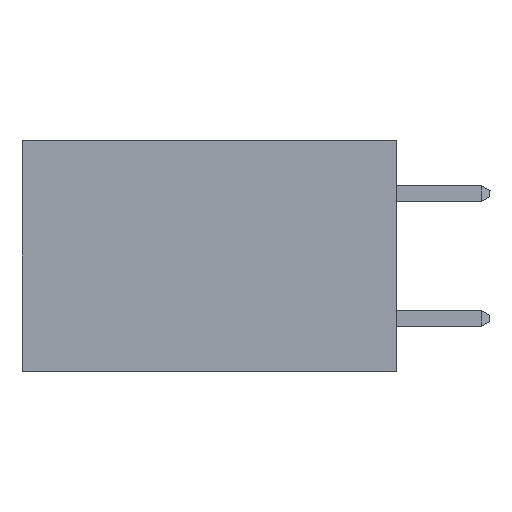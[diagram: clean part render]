
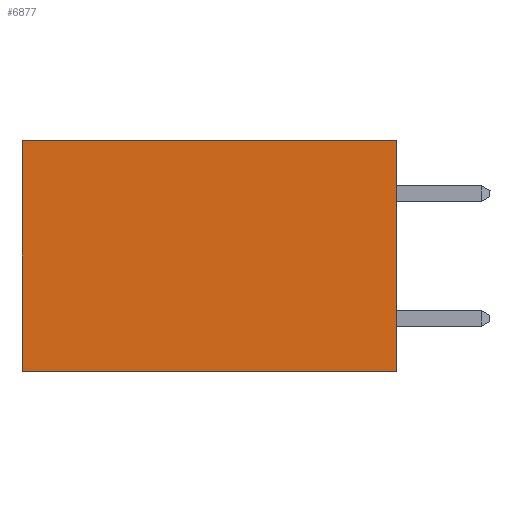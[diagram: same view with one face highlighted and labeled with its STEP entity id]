
A CAD part, left-side view. The second image highlights one B-rep face of the part: STEP entity #6877.
In plain terms, the highlighted planar face has unit normal (-1, 0, 0).
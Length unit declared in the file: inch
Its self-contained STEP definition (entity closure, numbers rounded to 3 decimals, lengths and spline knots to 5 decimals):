
#587 = VECTOR ( 'NONE', #7945, 39.37008 ) ;
#888 = CARTESIAN_POINT ( 'NONE',  ( 0.298, 0., 0. ) ) ;
#1716 = EDGE_CURVE ( 'NONE', #7474, #4993, #7250, .T. ) ;
#2394 = LINE ( 'NONE', #888, #11599 ) ;
#2653 = CARTESIAN_POINT ( 'NONE',  ( 0.298, 0.6, 0. ) ) ;
#3025 = ORIENTED_EDGE ( 'NONE', *, *, #7751, .F. ) ;
#4807 = LINE ( 'NONE', #15001, #8290 ) ;
#4993 = VERTEX_POINT ( 'NONE', #13291 ) ;
#5114 = ORIENTED_EDGE ( 'NONE', *, *, #14596, .F. ) ;
#5554 = DIRECTION ( 'NONE',  ( 0., 1., 0. ) ) ;
#6101 = VERTEX_POINT ( 'NONE', #13336 ) ;
#6487 = DIRECTION ( 'NONE',  ( 0., 1., 0. ) ) ;
#6577 = VERTEX_POINT ( 'NONE', #14257 ) ;
#6877 = ADVANCED_FACE ( 'NONE', ( #13568 ), #10319, .F. ) ;
#7250 = LINE ( 'NONE', #10048, #587 ) ;
#7474 = VERTEX_POINT ( 'NONE', #2653 ) ;
#7751 = EDGE_CURVE ( 'NONE', #6101, #4993, #9811, .T. ) ;
#7945 = DIRECTION ( 'NONE',  ( 0., 0., -1. ) ) ;
#8290 = VECTOR ( 'NONE', #6487, 39.37008 ) ;
#8355 = EDGE_CURVE ( 'NONE', #6577, #7474, #4807, .T. ) ;
#8827 = AXIS2_PLACEMENT_3D ( 'NONE', #10637, #10237, #10155 ) ;
#9141 = DIRECTION ( 'NONE',  ( 0., 0., -1. ) ) ;
#9811 = LINE ( 'NONE', #12825, #13152 ) ;
#10048 = CARTESIAN_POINT ( 'NONE',  ( 0.298, 0.6, 0. ) ) ;
#10155 = DIRECTION ( 'NONE',  ( 0., 0., -1. ) ) ;
#10237 = DIRECTION ( 'NONE',  ( 1., 0., 0. ) ) ;
#10319 = PLANE ( 'NONE',  #8827 ) ;
#10637 = CARTESIAN_POINT ( 'NONE',  ( 0.298, 0., 0. ) ) ;
#11599 = VECTOR ( 'NONE', #9141, 39.37008 ) ;
#12330 = ORIENTED_EDGE ( 'NONE', *, *, #1716, .T. ) ;
#12825 = CARTESIAN_POINT ( 'NONE',  ( 0.298, 0., -0.37 ) ) ;
#13152 = VECTOR ( 'NONE', #5554, 39.37008 ) ;
#13192 = ORIENTED_EDGE ( 'NONE', *, *, #8355, .T. ) ;
#13291 = CARTESIAN_POINT ( 'NONE',  ( 0.298, 0.6, -0.37 ) ) ;
#13336 = CARTESIAN_POINT ( 'NONE',  ( 0.298, 0., -0.37 ) ) ;
#13568 = FACE_OUTER_BOUND ( 'NONE', #15378, .T. ) ;
#14257 = CARTESIAN_POINT ( 'NONE',  ( 0.298, 0., 0. ) ) ;
#14596 = EDGE_CURVE ( 'NONE', #6577, #6101, #2394, .T. ) ;
#15001 = CARTESIAN_POINT ( 'NONE',  ( 0.298, 0., 0. ) ) ;
#15378 = EDGE_LOOP ( 'NONE', ( #12330, #3025, #5114, #13192 ) ) ;
